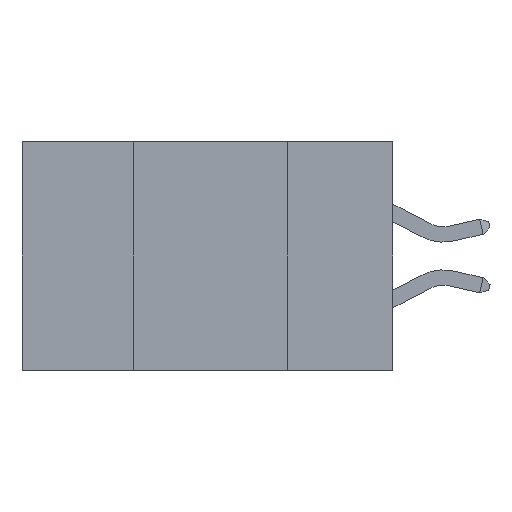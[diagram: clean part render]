
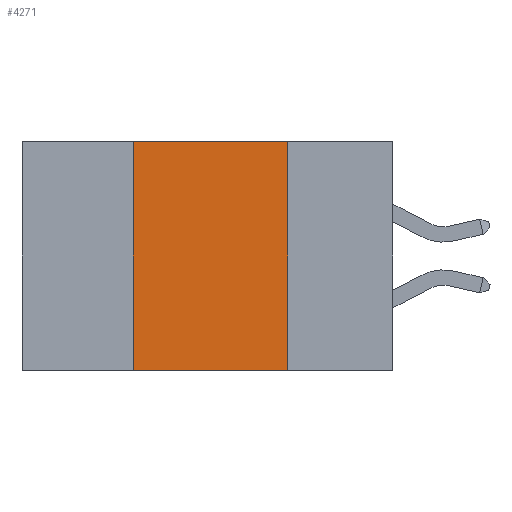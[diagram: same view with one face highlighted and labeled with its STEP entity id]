
A CAD part, left-side view. The second image highlights one B-rep face of the part: STEP entity #4271.
In plain terms, the highlighted planar face has unit normal (-1, 0, 0).
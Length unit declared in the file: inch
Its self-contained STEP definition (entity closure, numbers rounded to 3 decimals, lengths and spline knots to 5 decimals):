
#1284 = FACE_OUTER_BOUND ( 'NONE', #4776, .T. ) ;
#1361 = DIRECTION ( 'NONE',  ( 0., 0., -1. ) ) ;
#1716 = DIRECTION ( 'NONE',  ( 0., -1., 0. ) ) ;
#2350 = ORIENTED_EDGE ( 'NONE', *, *, #11509, .F. ) ;
#3425 = EDGE_CURVE ( 'NONE', #15021, #15167, #11104, .T. ) ;
#4271 = ADVANCED_FACE ( 'NONE', ( #1284 ), #5846, .F. ) ;
#4515 = CARTESIAN_POINT ( 'NONE',  ( 0., 0.17, 0. ) ) ;
#4776 = EDGE_LOOP ( 'NONE', ( #15463, #19266, #2350, #9510 ) ) ;
#5199 = CARTESIAN_POINT ( 'NONE',  ( 0., 0.17, 0. ) ) ;
#5832 = VERTEX_POINT ( 'NONE', #5199 ) ;
#5846 = PLANE ( 'NONE',  #17849 ) ;
#6419 = VECTOR ( 'NONE', #7892, 39.37008 ) ;
#6578 = VERTEX_POINT ( 'NONE', #10626 ) ;
#7053 = DIRECTION ( 'NONE',  ( 0., -1., 0. ) ) ;
#7401 = CARTESIAN_POINT ( 'NONE',  ( 0., 0.6, 0. ) ) ;
#7892 = DIRECTION ( 'NONE',  ( 0., 0., 1. ) ) ;
#8141 = LINE ( 'NONE', #4515, #8623 ) ;
#8623 = VECTOR ( 'NONE', #1361, 39.37008 ) ;
#9510 = ORIENTED_EDGE ( 'NONE', *, *, #3425, .T. ) ;
#10559 = CARTESIAN_POINT ( 'NONE',  ( 0., 0.42, 0. ) ) ;
#10626 = CARTESIAN_POINT ( 'NONE',  ( 0., 0.42, 0. ) ) ;
#11104 = LINE ( 'NONE', #17346, #19863 ) ;
#11509 = EDGE_CURVE ( 'NONE', #15021, #6578, #19041, .T. ) ;
#14217 = CARTESIAN_POINT ( 'NONE',  ( 0., 0.42, -0.37 ) ) ;
#14464 = VECTOR ( 'NONE', #7053, 39.37008 ) ;
#15021 = VERTEX_POINT ( 'NONE', #14217 ) ;
#15167 = VERTEX_POINT ( 'NONE', #17693 ) ;
#15463 = ORIENTED_EDGE ( 'NONE', *, *, #19044, .F. ) ;
#16901 = LINE ( 'NONE', #18788, #14464 ) ;
#17346 = CARTESIAN_POINT ( 'NONE',  ( 0., 0.6, -0.37 ) ) ;
#17693 = CARTESIAN_POINT ( 'NONE',  ( 0., 0.17, -0.37 ) ) ;
#17849 = AXIS2_PLACEMENT_3D ( 'NONE', #7401, #18271, #19871 ) ;
#17901 = EDGE_CURVE ( 'NONE', #6578, #5832, #16901, .T. ) ;
#18271 = DIRECTION ( 'NONE',  ( 1., 0., 0. ) ) ;
#18788 = CARTESIAN_POINT ( 'NONE',  ( 0., 0.6, 0. ) ) ;
#19041 = LINE ( 'NONE', #10559, #6419 ) ;
#19044 = EDGE_CURVE ( 'NONE', #5832, #15167, #8141, .T. ) ;
#19266 = ORIENTED_EDGE ( 'NONE', *, *, #17901, .F. ) ;
#19863 = VECTOR ( 'NONE', #1716, 39.37008 ) ;
#19871 = DIRECTION ( 'NONE',  ( 0., 0., -1. ) ) ;
